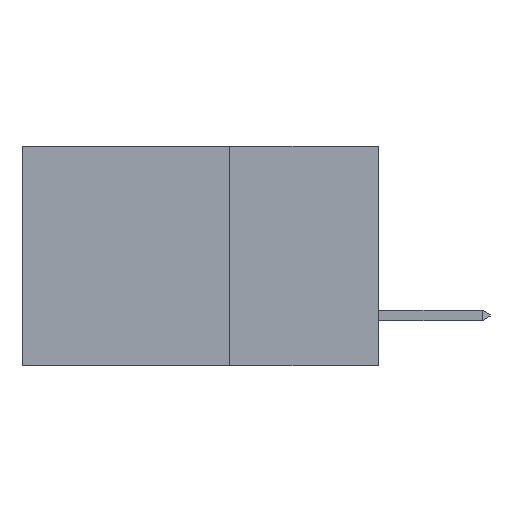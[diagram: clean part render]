
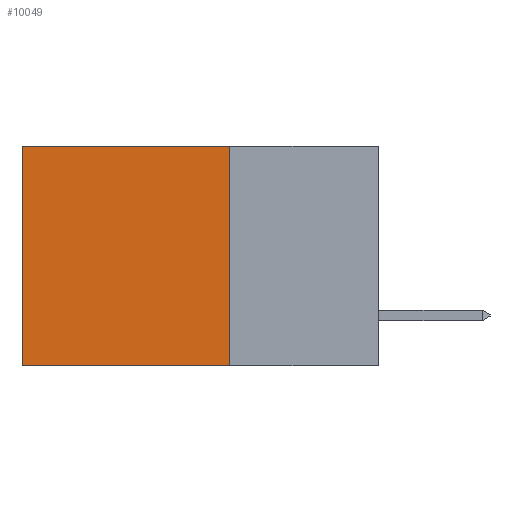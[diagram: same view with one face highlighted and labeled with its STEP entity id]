
A CAD part, left-side view. The second image highlights one B-rep face of the part: STEP entity #10049.
In plain terms, the highlighted planar face has unit normal (-1, 0, 0).
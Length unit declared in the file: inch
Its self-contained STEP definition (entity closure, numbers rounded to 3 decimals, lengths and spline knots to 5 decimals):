
#63 = CARTESIAN_POINT ( 'NONE',  ( 0.2615, 0.25, 0. ) ) ;
#340 = EDGE_CURVE ( 'NONE', #1230, #7730, #5615, .T. ) ;
#488 = VERTEX_POINT ( 'NONE', #7742 ) ;
#697 = CARTESIAN_POINT ( 'NONE',  ( 0.2615, 0.25, -0.37 ) ) ;
#1230 = VERTEX_POINT ( 'NONE', #63 ) ;
#1259 = VECTOR ( 'NONE', #2847, 39.37008 ) ;
#1631 = LINE ( 'NONE', #3208, #5973 ) ;
#2304 = DIRECTION ( 'NONE',  ( 0., 1., 0. ) ) ;
#2769 = DIRECTION ( 'NONE',  ( 0., 0., -1. ) ) ;
#2847 = DIRECTION ( 'NONE',  ( 0., 1., 0. ) ) ;
#2955 = DIRECTION ( 'NONE',  ( 1., 0., 0. ) ) ;
#3208 = CARTESIAN_POINT ( 'NONE',  ( 0.2615, 0.25, -0.37 ) ) ;
#3656 = EDGE_CURVE ( 'NONE', #7730, #488, #7158, .T. ) ;
#3797 = LINE ( 'NONE', #7922, #10286 ) ;
#3966 = EDGE_CURVE ( 'NONE', #10375, #488, #1631, .T. ) ;
#4185 = EDGE_CURVE ( 'NONE', #1230, #10375, #3797, .T. ) ;
#4193 = ORIENTED_EDGE ( 'NONE', *, *, #3966, .F. ) ;
#4453 = ORIENTED_EDGE ( 'NONE', *, *, #4185, .F. ) ;
#4737 = ORIENTED_EDGE ( 'NONE', *, *, #340, .T. ) ;
#4916 = VECTOR ( 'NONE', #2769, 39.37008 ) ;
#5048 = EDGE_LOOP ( 'NONE', ( #10668, #4193, #4453, #4737 ) ) ;
#5615 = LINE ( 'NONE', #10963, #1259 ) ;
#5973 = VECTOR ( 'NONE', #2304, 39.37008 ) ;
#6410 = PLANE ( 'NONE',  #7054 ) ;
#6423 = CARTESIAN_POINT ( 'NONE',  ( 0.2615, 0.6, 0. ) ) ;
#7054 = AXIS2_PLACEMENT_3D ( 'NONE', #8058, #2955, #8899 ) ;
#7158 = LINE ( 'NONE', #7898, #4916 ) ;
#7730 = VERTEX_POINT ( 'NONE', #6423 ) ;
#7742 = CARTESIAN_POINT ( 'NONE',  ( 0.2615, 0.6, -0.37 ) ) ;
#7898 = CARTESIAN_POINT ( 'NONE',  ( 0.2615, 0.6, -0.37 ) ) ;
#7922 = CARTESIAN_POINT ( 'NONE',  ( 0.2615, 0.25, -0.37 ) ) ;
#7994 = FACE_OUTER_BOUND ( 'NONE', #5048, .T. ) ;
#8058 = CARTESIAN_POINT ( 'NONE',  ( 0.2615, 0.25, -0.37 ) ) ;
#8747 = DIRECTION ( 'NONE',  ( 0., 0., -1. ) ) ;
#8899 = DIRECTION ( 'NONE',  ( 0., 0., -1. ) ) ;
#10049 = ADVANCED_FACE ( 'NONE', ( #7994 ), #6410, .F. ) ;
#10286 = VECTOR ( 'NONE', #8747, 39.37008 ) ;
#10375 = VERTEX_POINT ( 'NONE', #697 ) ;
#10668 = ORIENTED_EDGE ( 'NONE', *, *, #3656, .T. ) ;
#10963 = CARTESIAN_POINT ( 'NONE',  ( 0.2615, 0.25, 0. ) ) ;
